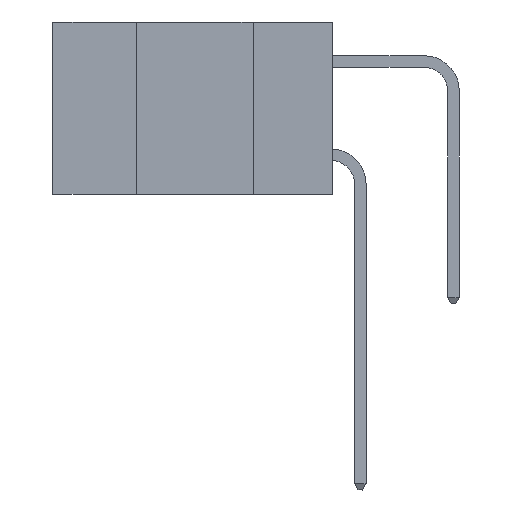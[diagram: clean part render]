
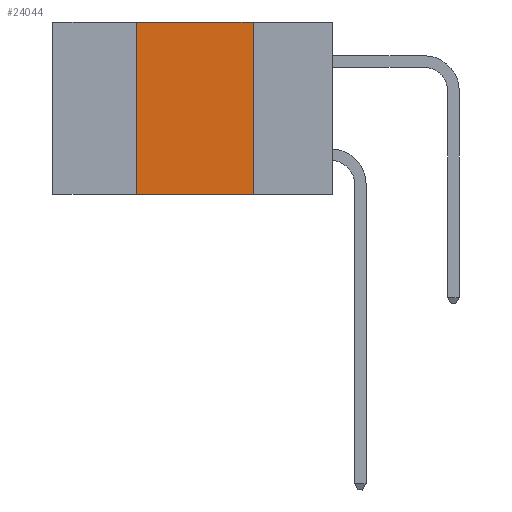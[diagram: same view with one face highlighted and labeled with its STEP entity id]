
A CAD part, left-side view. The second image highlights one B-rep face of the part: STEP entity #24044.
In plain terms, the highlighted planar face has unit normal (-1, 0, 0).
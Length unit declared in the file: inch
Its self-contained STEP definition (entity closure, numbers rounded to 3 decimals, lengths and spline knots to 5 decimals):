
#889 = VERTEX_POINT ( 'NONE', #1872 ) ;
#1872 = CARTESIAN_POINT ( 'NONE',  ( 0., 0.42, 0. ) ) ;
#2318 = EDGE_CURVE ( 'NONE', #7660, #8359, #23376, .T. ) ;
#2475 = ORIENTED_EDGE ( 'NONE', *, *, #5775, .F. ) ;
#5184 = DIRECTION ( 'NONE',  ( 0., 0., 1. ) ) ;
#5775 = EDGE_CURVE ( 'NONE', #31356, #8359, #28254, .T. ) ;
#6146 = CARTESIAN_POINT ( 'NONE',  ( 0., 0.6, -0.37 ) ) ;
#6852 = FACE_OUTER_BOUND ( 'NONE', #18980, .T. ) ;
#7660 = VERTEX_POINT ( 'NONE', #32995 ) ;
#7901 = VECTOR ( 'NONE', #33829, 39.37008 ) ;
#8359 = VERTEX_POINT ( 'NONE', #26267 ) ;
#10083 = LINE ( 'NONE', #32095, #29246 ) ;
#11130 = EDGE_CURVE ( 'NONE', #889, #31356, #30806, .T. ) ;
#11306 = DIRECTION ( 'NONE',  ( 0., 0., -1. ) ) ;
#12814 = CARTESIAN_POINT ( 'NONE',  ( 0., 0.6, 0. ) ) ;
#13842 = PLANE ( 'NONE',  #27540 ) ;
#14041 = CARTESIAN_POINT ( 'NONE',  ( 0., 0.17, 0. ) ) ;
#14850 = EDGE_CURVE ( 'NONE', #7660, #889, #10083, .T. ) ;
#18980 = EDGE_LOOP ( 'NONE', ( #2475, #22443, #24117, #29952 ) ) ;
#19759 = DIRECTION ( 'NONE',  ( 0., -1., 0. ) ) ;
#22443 = ORIENTED_EDGE ( 'NONE', *, *, #11130, .F. ) ;
#23260 = VECTOR ( 'NONE', #33173, 39.37008 ) ;
#23376 = LINE ( 'NONE', #6146, #27111 ) ;
#24044 = ADVANCED_FACE ( 'NONE', ( #6852 ), #13842, .F. ) ;
#24117 = ORIENTED_EDGE ( 'NONE', *, *, #14850, .F. ) ;
#25117 = CARTESIAN_POINT ( 'NONE',  ( 0., 0.17, 0. ) ) ;
#26267 = CARTESIAN_POINT ( 'NONE',  ( 0., 0.17, -0.37 ) ) ;
#27029 = DIRECTION ( 'NONE',  ( 1., 0., 0. ) ) ;
#27111 = VECTOR ( 'NONE', #19759, 39.37008 ) ;
#27148 = CARTESIAN_POINT ( 'NONE',  ( 0., 0.6, 0. ) ) ;
#27540 = AXIS2_PLACEMENT_3D ( 'NONE', #27148, #27029, #11306 ) ;
#28254 = LINE ( 'NONE', #14041, #23260 ) ;
#29246 = VECTOR ( 'NONE', #5184, 39.37008 ) ;
#29952 = ORIENTED_EDGE ( 'NONE', *, *, #2318, .T. ) ;
#30806 = LINE ( 'NONE', #12814, #7901 ) ;
#31356 = VERTEX_POINT ( 'NONE', #25117 ) ;
#32095 = CARTESIAN_POINT ( 'NONE',  ( 0., 0.42, 0. ) ) ;
#32995 = CARTESIAN_POINT ( 'NONE',  ( 0., 0.42, -0.37 ) ) ;
#33173 = DIRECTION ( 'NONE',  ( 0., 0., -1. ) ) ;
#33829 = DIRECTION ( 'NONE',  ( 0., -1., 0. ) ) ;
